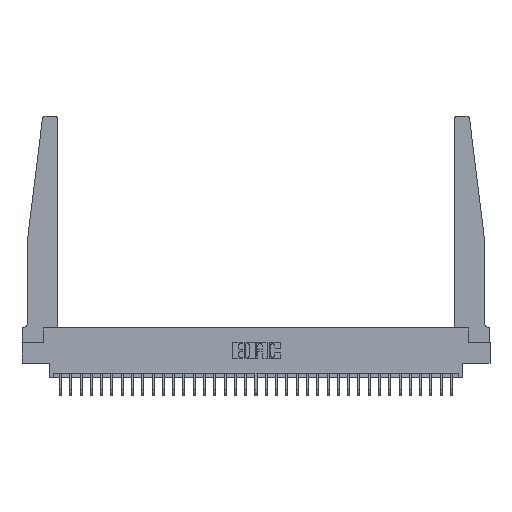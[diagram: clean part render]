
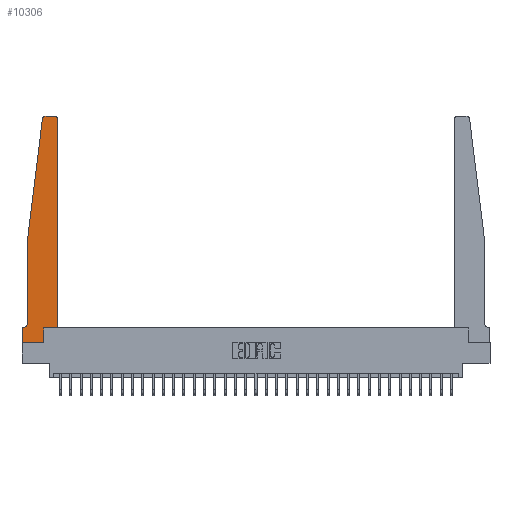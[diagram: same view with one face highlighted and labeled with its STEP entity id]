
A CAD part, top view. The second image highlights one B-rep face of the part: STEP entity #10306.
In plain terms, the highlighted planar face has unit normal (0, 0, 1).
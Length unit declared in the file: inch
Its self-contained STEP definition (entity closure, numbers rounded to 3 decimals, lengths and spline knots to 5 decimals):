
#166 = DIRECTION ( 'NONE',  ( 0., 1., 0. ) ) ;
#648 = CIRCLE ( 'NONE', #4965, 0.03 ) ;
#884 = VERTEX_POINT ( 'NONE', #20433 ) ;
#1740 = AXIS2_PLACEMENT_3D ( 'NONE', #12201, #12042, #7054 ) ;
#2018 = CARTESIAN_POINT ( 'NONE',  ( 0.425, 0.18, 0.37 ) ) ;
#2351 = LINE ( 'NONE', #15523, #5794 ) ;
#2789 = VERTEX_POINT ( 'NONE', #12347 ) ;
#3483 = ORIENTED_EDGE ( 'NONE', *, *, #18265, .T. ) ;
#3894 = ORIENTED_EDGE ( 'NONE', *, *, #31540, .T. ) ;
#4143 = CARTESIAN_POINT ( 'NONE',  ( 0.24675, 2.72367, 0.37 ) ) ;
#4499 = CARTESIAN_POINT ( 'NONE',  ( 0., 0., 0.37 ) ) ;
#4504 = CARTESIAN_POINT ( 'NONE',  ( 0., 0.1875, 0.37 ) ) ;
#4763 = VERTEX_POINT ( 'NONE', #20079 ) ;
#4965 = AXIS2_PLACEMENT_3D ( 'NONE', #26023, #8202, #13350 ) ;
#5278 = CARTESIAN_POINT ( 'NONE',  ( 0., 0., 0.37 ) ) ;
#5794 = VECTOR ( 'NONE', #166, 39.37008 ) ;
#6555 = CIRCLE ( 'NONE', #1740, 0.03 ) ;
#6652 = ORIENTED_EDGE ( 'NONE', *, *, #26777, .T. ) ;
#6830 = VECTOR ( 'NONE', #17050, 39.37008 ) ;
#6998 = VECTOR ( 'NONE', #28370, 39.37008 ) ;
#7054 = DIRECTION ( 'NONE',  ( 1., 0., 0. ) ) ;
#7572 = AXIS2_PLACEMENT_3D ( 'NONE', #16293, #11459, #23970 ) ;
#7694 = PLANE ( 'NONE',  #18297 ) ;
#7928 = VERTEX_POINT ( 'NONE', #19006 ) ;
#7992 = CARTESIAN_POINT ( 'NONE',  ( 0.065, 1.25, 0.37 ) ) ;
#8070 = VERTEX_POINT ( 'NONE', #4143 ) ;
#8169 = CARTESIAN_POINT ( 'NONE',  ( 0.015, 0.1875, 0.37 ) ) ;
#8202 = DIRECTION ( 'NONE',  ( 0., 0., 1. ) ) ;
#8273 = VERTEX_POINT ( 'NONE', #8169 ) ;
#8317 = DIRECTION ( 'NONE',  ( 0., -1., 0. ) ) ;
#9666 = CIRCLE ( 'NONE', #7572, 0.05 ) ;
#10303 = DIRECTION ( 'NONE',  ( 1., 0., 0. ) ) ;
#10306 = ADVANCED_FACE ( 'NONE', ( #25704 ), #7694, .T. ) ;
#10459 = LINE ( 'NONE', #5278, #24843 ) ;
#10613 = ORIENTED_EDGE ( 'NONE', *, *, #32758, .T. ) ;
#10631 = VERTEX_POINT ( 'NONE', #22151 ) ;
#10783 = LINE ( 'NONE', #18437, #24645 ) ;
#11459 = DIRECTION ( 'NONE',  ( 0., 0., -1. ) ) ;
#12042 = DIRECTION ( 'NONE',  ( 0., 0., 1. ) ) ;
#12051 = LINE ( 'NONE', #27577, #6830 ) ;
#12185 = CARTESIAN_POINT ( 'NONE',  ( 0., 0.1875, 0.37 ) ) ;
#12201 = CARTESIAN_POINT ( 'NONE',  ( 0.27653, 2.72, 0.37 ) ) ;
#12347 = CARTESIAN_POINT ( 'NONE',  ( 0.065, 0.2375, 0.37 ) ) ;
#13350 = DIRECTION ( 'NONE',  ( 1., 0., 0. ) ) ;
#14812 = LINE ( 'NONE', #32715, #20564 ) ;
#14833 = VECTOR ( 'NONE', #25268, 39.37008 ) ;
#15072 = CARTESIAN_POINT ( 'NONE',  ( 0.065, 1.25, 0.37 ) ) ;
#15489 = EDGE_CURVE ( 'NONE', #10631, #884, #10783, .T. ) ;
#15523 = CARTESIAN_POINT ( 'NONE',  ( 0.2605, 0.18, 0.37 ) ) ;
#15706 = ORIENTED_EDGE ( 'NONE', *, *, #16232, .T. ) ;
#15972 = LINE ( 'NONE', #7992, #19884 ) ;
#16133 = VERTEX_POINT ( 'NONE', #2018 ) ;
#16232 = EDGE_CURVE ( 'NONE', #884, #8070, #6555, .T. ) ;
#16293 = CARTESIAN_POINT ( 'NONE',  ( 0.015, 0.2375, 0.37 ) ) ;
#16431 = EDGE_CURVE ( 'NONE', #29872, #2789, #15972, .T. ) ;
#17050 = DIRECTION ( 'NONE',  ( -1., 0., 0. ) ) ;
#17706 = EDGE_CURVE ( 'NONE', #31237, #18949, #14812, .T. ) ;
#18117 = DIRECTION ( 'NONE',  ( -1., 0., 0. ) ) ;
#18265 = EDGE_CURVE ( 'NONE', #18949, #7928, #10459, .T. ) ;
#18297 = AXIS2_PLACEMENT_3D ( 'NONE', #4504, #25525, #20521 ) ;
#18437 = CARTESIAN_POINT ( 'NONE',  ( 0.25, 2.75, 0.37 ) ) ;
#18949 = VERTEX_POINT ( 'NONE', #4499 ) ;
#19006 = CARTESIAN_POINT ( 'NONE',  ( 0.2605, 0., 0.37 ) ) ;
#19157 = CARTESIAN_POINT ( 'NONE',  ( 0.065, 1.25, 0.37 ) ) ;
#19842 = DIRECTION ( 'NONE',  ( 0., -1., 0. ) ) ;
#19884 = VECTOR ( 'NONE', #8317, 39.37008 ) ;
#20079 = CARTESIAN_POINT ( 'NONE',  ( 0.2605, 0.18, 0.37 ) ) ;
#20110 = DIRECTION ( 'NONE',  ( 0., 1., 0. ) ) ;
#20385 = EDGE_CURVE ( 'NONE', #8273, #31237, #12051, .T. ) ;
#20433 = CARTESIAN_POINT ( 'NONE',  ( 0.27653, 2.75, 0.37 ) ) ;
#20457 = ORIENTED_EDGE ( 'NONE', *, *, #23729, .T. ) ;
#20521 = DIRECTION ( 'NONE',  ( 1., 0., 0. ) ) ;
#20564 = VECTOR ( 'NONE', #19842, 39.37008 ) ;
#21360 = VERTEX_POINT ( 'NONE', #22435 ) ;
#22151 = CARTESIAN_POINT ( 'NONE',  ( 0.395, 2.75, 0.37 ) ) ;
#22435 = CARTESIAN_POINT ( 'NONE',  ( 0.425, 2.72, 0.37 ) ) ;
#22784 = ORIENTED_EDGE ( 'NONE', *, *, #25812, .T. ) ;
#23729 = EDGE_CURVE ( 'NONE', #4763, #16133, #30698, .T. ) ;
#23869 = EDGE_LOOP ( 'NONE', ( #27267, #15706, #23920, #30859, #3894, #24000, #27993, #3483, #6652, #20457, #22784, #10613 ) ) ;
#23920 = ORIENTED_EDGE ( 'NONE', *, *, #26395, .T. ) ;
#23970 = DIRECTION ( 'NONE',  ( -1., 0., 0. ) ) ;
#24000 = ORIENTED_EDGE ( 'NONE', *, *, #20385, .T. ) ;
#24419 = VECTOR ( 'NONE', #20110, 39.37008 ) ;
#24645 = VECTOR ( 'NONE', #18117, 39.37008 ) ;
#24843 = VECTOR ( 'NONE', #10303, 39.37008 ) ;
#25136 = LINE ( 'NONE', #27303, #24419 ) ;
#25268 = DIRECTION ( 'NONE',  ( -0.122, -0.992, 0. ) ) ;
#25525 = DIRECTION ( 'NONE',  ( 0., 0., 1. ) ) ;
#25704 = FACE_OUTER_BOUND ( 'NONE', #23869, .T. ) ;
#25812 = EDGE_CURVE ( 'NONE', #16133, #21360, #25136, .T. ) ;
#26023 = CARTESIAN_POINT ( 'NONE',  ( 0.395, 2.72, 0.37 ) ) ;
#26395 = EDGE_CURVE ( 'NONE', #8070, #29872, #32780, .T. ) ;
#26777 = EDGE_CURVE ( 'NONE', #7928, #4763, #2351, .T. ) ;
#27267 = ORIENTED_EDGE ( 'NONE', *, *, #15489, .T. ) ;
#27303 = CARTESIAN_POINT ( 'NONE',  ( 0.425, 0.18, 0.37 ) ) ;
#27577 = CARTESIAN_POINT ( 'NONE',  ( 0.065, 0.1875, 0.37 ) ) ;
#27706 = CARTESIAN_POINT ( 'NONE',  ( 0.425, 0.18, 0.37 ) ) ;
#27993 = ORIENTED_EDGE ( 'NONE', *, *, #17706, .T. ) ;
#28370 = DIRECTION ( 'NONE',  ( 1., 0., 0. ) ) ;
#29872 = VERTEX_POINT ( 'NONE', #19157 ) ;
#30698 = LINE ( 'NONE', #27706, #6998 ) ;
#30859 = ORIENTED_EDGE ( 'NONE', *, *, #16431, .T. ) ;
#31237 = VERTEX_POINT ( 'NONE', #12185 ) ;
#31540 = EDGE_CURVE ( 'NONE', #2789, #8273, #9666, .T. ) ;
#32715 = CARTESIAN_POINT ( 'NONE',  ( 0., 0., 0.37 ) ) ;
#32758 = EDGE_CURVE ( 'NONE', #21360, #10631, #648, .T. ) ;
#32780 = LINE ( 'NONE', #15072, #14833 ) ;
